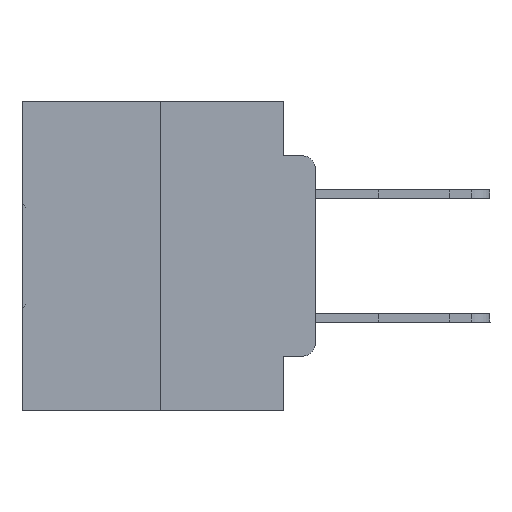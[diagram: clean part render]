
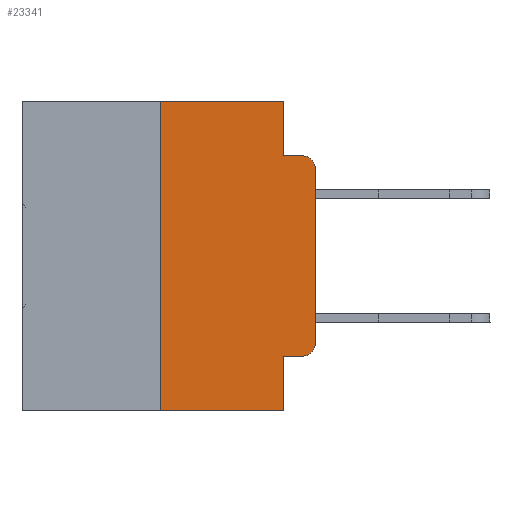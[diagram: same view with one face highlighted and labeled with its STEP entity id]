
A CAD part, left-side view. The second image highlights one B-rep face of the part: STEP entity #23341.
In plain terms, the highlighted planar face has unit normal (-1, 0, 0).
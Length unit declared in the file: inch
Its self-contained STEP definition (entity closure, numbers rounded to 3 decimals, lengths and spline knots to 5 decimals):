
#39 = ORIENTED_EDGE ( 'NONE', *, *, #7644, .T. ) ;
#685 = DIRECTION ( 'NONE',  ( 0., -1., 0. ) ) ;
#1804 = CARTESIAN_POINT ( 'NONE',  ( 0., 0.25, 0. ) ) ;
#2809 = ORIENTED_EDGE ( 'NONE', *, *, #3408, .F. ) ;
#3098 = VERTEX_POINT ( 'NONE', #28965 ) ;
#3118 = ORIENTED_EDGE ( 'NONE', *, *, #11082, .T. ) ;
#3264 = DIRECTION ( 'NONE',  ( 0., 0., 1. ) ) ;
#3383 = ORIENTED_EDGE ( 'NONE', *, *, #6978, .F. ) ;
#3408 = EDGE_CURVE ( 'NONE', #33125, #18575, #17003, .T. ) ;
#3669 = CARTESIAN_POINT ( 'NONE',  ( 0., 0.051, -0.5 ) ) ;
#4565 = EDGE_CURVE ( 'NONE', #12358, #17524, #29183, .T. ) ;
#4864 = CARTESIAN_POINT ( 'NONE',  ( 0., 0.051, -0.0885 ) ) ;
#6518 = DIRECTION ( 'NONE',  ( 0., 0., -1. ) ) ;
#6851 = ORIENTED_EDGE ( 'NONE', *, *, #29808, .T. ) ;
#6968 = CARTESIAN_POINT ( 'NONE',  ( 0., 0.25, -0.5 ) ) ;
#6978 = EDGE_CURVE ( 'NONE', #18575, #26023, #20099, .T. ) ;
#7044 = DIRECTION ( 'NONE',  ( 0., 0., -1. ) ) ;
#7101 = AXIS2_PLACEMENT_3D ( 'NONE', #19517, #32177, #19396 ) ;
#7644 = EDGE_CURVE ( 'NONE', #18564, #3098, #13901, .T. ) ;
#8188 = ORIENTED_EDGE ( 'NONE', *, *, #32550, .F. ) ;
#8355 = LINE ( 'NONE', #18976, #20671 ) ;
#8785 = CARTESIAN_POINT ( 'NONE',  ( 0., 0.25, 0. ) ) ;
#8788 = ORIENTED_EDGE ( 'NONE', *, *, #4565, .T. ) ;
#9478 = VECTOR ( 'NONE', #19114, 39.37008 ) ;
#9658 = VECTOR ( 'NONE', #28737, 39.37008 ) ;
#9716 = VECTOR ( 'NONE', #27077, 39.37008 ) ;
#10483 = LINE ( 'NONE', #33767, #9658 ) ;
#10550 = VERTEX_POINT ( 'NONE', #3669 ) ;
#11082 = EDGE_CURVE ( 'NONE', #3098, #29080, #22427, .T. ) ;
#12134 = VECTOR ( 'NONE', #12291, 39.37008 ) ;
#12291 = DIRECTION ( 'NONE',  ( 0., 0., 1. ) ) ;
#12358 = VERTEX_POINT ( 'NONE', #15882 ) ;
#12462 = CARTESIAN_POINT ( 'NONE',  ( 0., 0.051, -0.4115 ) ) ;
#12613 = ORIENTED_EDGE ( 'NONE', *, *, #14996, .F. ) ;
#13901 = LINE ( 'NONE', #12462, #20848 ) ;
#14403 = EDGE_CURVE ( 'NONE', #33788, #17524, #29147, .T. ) ;
#14681 = CARTESIAN_POINT ( 'NONE',  ( 0., 0.473, 0. ) ) ;
#14996 = EDGE_CURVE ( 'NONE', #18564, #10550, #16821, .T. ) ;
#15271 = VECTOR ( 'NONE', #685, 39.37008 ) ;
#15882 = CARTESIAN_POINT ( 'NONE',  ( 0., 0., -0.1085 ) ) ;
#16333 = CARTESIAN_POINT ( 'NONE',  ( 0., 0.473, 0. ) ) ;
#16651 = CARTESIAN_POINT ( 'NONE',  ( 0., 0.051, -0.0885 ) ) ;
#16724 = DIRECTION ( 'NONE',  ( 1., 0., 0. ) ) ;
#16821 = LINE ( 'NONE', #21631, #9478 ) ;
#17003 = LINE ( 'NONE', #1804, #12134 ) ;
#17524 = VERTEX_POINT ( 'NONE', #25462 ) ;
#17891 = DIRECTION ( 'NONE',  ( 0., -1., 0. ) ) ;
#18537 = ORIENTED_EDGE ( 'NONE', *, *, #25823, .T. ) ;
#18564 = VERTEX_POINT ( 'NONE', #32225 ) ;
#18575 = VERTEX_POINT ( 'NONE', #8785 ) ;
#18976 = CARTESIAN_POINT ( 'NONE',  ( 0., 0., 0. ) ) ;
#19114 = DIRECTION ( 'NONE',  ( 0., 0., -1. ) ) ;
#19362 = PLANE ( 'NONE',  #19607 ) ;
#19396 = DIRECTION ( 'NONE',  ( 0., 0., -1. ) ) ;
#19517 = CARTESIAN_POINT ( 'NONE',  ( 0., 0.02, -0.1085 ) ) ;
#19607 = AXIS2_PLACEMENT_3D ( 'NONE', #14681, #16724, #6518 ) ;
#20099 = LINE ( 'NONE', #16333, #9716 ) ;
#20104 = CARTESIAN_POINT ( 'NONE',  ( 0., 0.02, -0.3915 ) ) ;
#20671 = VECTOR ( 'NONE', #3264, 39.37008 ) ;
#20848 = VECTOR ( 'NONE', #17891, 39.37008 ) ;
#20880 = CARTESIAN_POINT ( 'NONE',  ( 0., 0.473, -0.5 ) ) ;
#21631 = CARTESIAN_POINT ( 'NONE',  ( 0., 0.051, 0. ) ) ;
#22427 = CIRCLE ( 'NONE', #30832, 0.02 ) ;
#22806 = ORIENTED_EDGE ( 'NONE', *, *, #14403, .F. ) ;
#22953 = CARTESIAN_POINT ( 'NONE',  ( 0., 0.051, 0. ) ) ;
#23341 = ADVANCED_FACE ( 'NONE', ( #25765 ), #19362, .F. ) ;
#23931 = DIRECTION ( 'NONE',  ( 0., -1., 0. ) ) ;
#24474 = CARTESIAN_POINT ( 'NONE',  ( 0., 0., -0.3915 ) ) ;
#25138 = DIRECTION ( 'NONE',  ( -1., 0., 0. ) ) ;
#25462 = CARTESIAN_POINT ( 'NONE',  ( 0., 0.02, -0.0885 ) ) ;
#25765 = FACE_OUTER_BOUND ( 'NONE', #32529, .T. ) ;
#25823 = EDGE_CURVE ( 'NONE', #29080, #12358, #8355, .T. ) ;
#26023 = VERTEX_POINT ( 'NONE', #22953 ) ;
#27077 = DIRECTION ( 'NONE',  ( 0., -1., 0. ) ) ;
#27879 = LINE ( 'NONE', #20880, #29890 ) ;
#28737 = DIRECTION ( 'NONE',  ( 0., 0., -1. ) ) ;
#28965 = CARTESIAN_POINT ( 'NONE',  ( 0., 0.02, -0.4115 ) ) ;
#29080 = VERTEX_POINT ( 'NONE', #24474 ) ;
#29147 = LINE ( 'NONE', #16651, #15271 ) ;
#29183 = CIRCLE ( 'NONE', #7101, 0.02 ) ;
#29808 = EDGE_CURVE ( 'NONE', #33125, #10550, #27879, .T. ) ;
#29890 = VECTOR ( 'NONE', #23931, 39.37008 ) ;
#30832 = AXIS2_PLACEMENT_3D ( 'NONE', #20104, #25138, #7044 ) ;
#32177 = DIRECTION ( 'NONE',  ( -1., 0., 0. ) ) ;
#32225 = CARTESIAN_POINT ( 'NONE',  ( 0., 0.051, -0.4115 ) ) ;
#32529 = EDGE_LOOP ( 'NONE', ( #18537, #8788, #22806, #8188, #3383, #2809, #6851, #12613, #39, #3118 ) ) ;
#32550 = EDGE_CURVE ( 'NONE', #26023, #33788, #10483, .T. ) ;
#33125 = VERTEX_POINT ( 'NONE', #6968 ) ;
#33767 = CARTESIAN_POINT ( 'NONE',  ( 0., 0.051, 0. ) ) ;
#33788 = VERTEX_POINT ( 'NONE', #4864 ) ;
